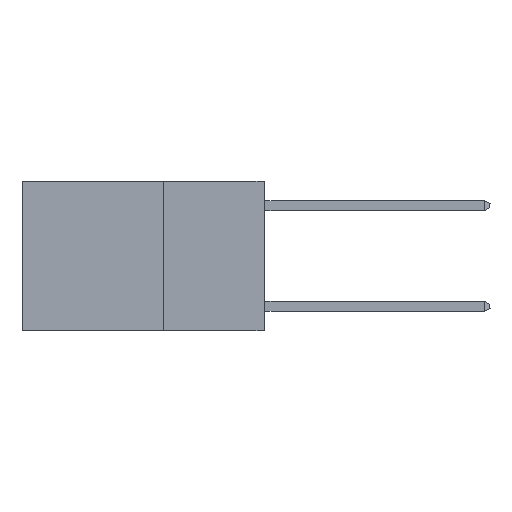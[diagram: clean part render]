
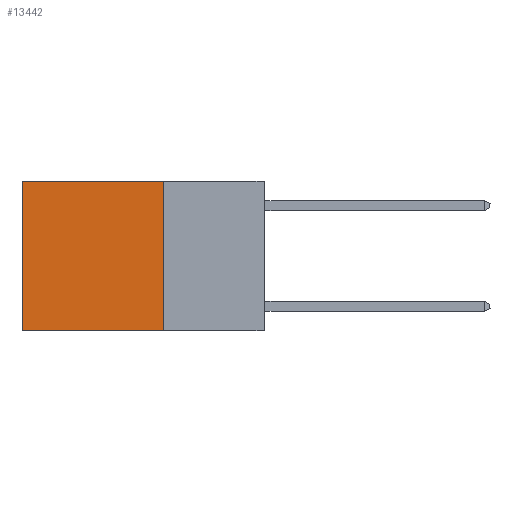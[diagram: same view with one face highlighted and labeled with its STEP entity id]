
A CAD part, left-side view. The second image highlights one B-rep face of the part: STEP entity #13442.
In plain terms, the highlighted planar face has unit normal (-1, 0, 0).
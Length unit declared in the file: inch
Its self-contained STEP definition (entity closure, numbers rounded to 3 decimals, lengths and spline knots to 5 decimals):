
#200 = ORIENTED_EDGE ( 'NONE', *, *, #17764, .F. ) ;
#1829 = EDGE_CURVE ( 'NONE', #8045, #3951, #3650, .T. ) ;
#2445 = CARTESIAN_POINT ( 'NONE',  ( 0.2625, 0.25, 0. ) ) ;
#2872 = VERTEX_POINT ( 'NONE', #17483 ) ;
#3065 = LINE ( 'NONE', #11735, #5301 ) ;
#3260 = CARTESIAN_POINT ( 'NONE',  ( 0.2625, 0.6, 0. ) ) ;
#3650 = LINE ( 'NONE', #2445, #4056 ) ;
#3951 = VERTEX_POINT ( 'NONE', #18074 ) ;
#4056 = VECTOR ( 'NONE', #20236, 39.37008 ) ;
#5115 = DIRECTION ( 'NONE',  ( 0., 0., -1. ) ) ;
#5301 = VECTOR ( 'NONE', #8049, 39.37008 ) ;
#7319 = DIRECTION ( 'NONE',  ( 1., 0., 0. ) ) ;
#8045 = VERTEX_POINT ( 'NONE', #20336 ) ;
#8049 = DIRECTION ( 'NONE',  ( 0., 0., -1. ) ) ;
#9985 = AXIS2_PLACEMENT_3D ( 'NONE', #15520, #7319, #20451 ) ;
#10124 = ORIENTED_EDGE ( 'NONE', *, *, #20081, .F. ) ;
#10126 = CARTESIAN_POINT ( 'NONE',  ( 0.2625, 0.6, -0.37 ) ) ;
#10620 = DIRECTION ( 'NONE',  ( 0., 1., 0. ) ) ;
#11735 = CARTESIAN_POINT ( 'NONE',  ( 0.2625, 0.25, 0. ) ) ;
#12245 = CARTESIAN_POINT ( 'NONE',  ( 0.2625, 0.25, -0.37 ) ) ;
#13134 = VECTOR ( 'NONE', #5115, 39.37008 ) ;
#13442 = ADVANCED_FACE ( 'NONE', ( #19053 ), #18846, .F. ) ;
#13633 = LINE ( 'NONE', #12245, #16939 ) ;
#14403 = EDGE_LOOP ( 'NONE', ( #16437, #200, #10124, #20736 ) ) ;
#14950 = LINE ( 'NONE', #3260, #13134 ) ;
#15520 = CARTESIAN_POINT ( 'NONE',  ( 0.2625, 0.25, 0. ) ) ;
#16437 = ORIENTED_EDGE ( 'NONE', *, *, #17621, .T. ) ;
#16939 = VECTOR ( 'NONE', #10620, 39.37008 ) ;
#17483 = CARTESIAN_POINT ( 'NONE',  ( 0.2625, 0.25, -0.37 ) ) ;
#17621 = EDGE_CURVE ( 'NONE', #3951, #20654, #14950, .T. ) ;
#17764 = EDGE_CURVE ( 'NONE', #2872, #20654, #13633, .T. ) ;
#18074 = CARTESIAN_POINT ( 'NONE',  ( 0.2625, 0.6, 0. ) ) ;
#18846 = PLANE ( 'NONE',  #9985 ) ;
#19053 = FACE_OUTER_BOUND ( 'NONE', #14403, .T. ) ;
#20081 = EDGE_CURVE ( 'NONE', #8045, #2872, #3065, .T. ) ;
#20236 = DIRECTION ( 'NONE',  ( 0., 1., 0. ) ) ;
#20336 = CARTESIAN_POINT ( 'NONE',  ( 0.2625, 0.25, 0. ) ) ;
#20451 = DIRECTION ( 'NONE',  ( 0., 0., -1. ) ) ;
#20654 = VERTEX_POINT ( 'NONE', #10126 ) ;
#20736 = ORIENTED_EDGE ( 'NONE', *, *, #1829, .T. ) ;
